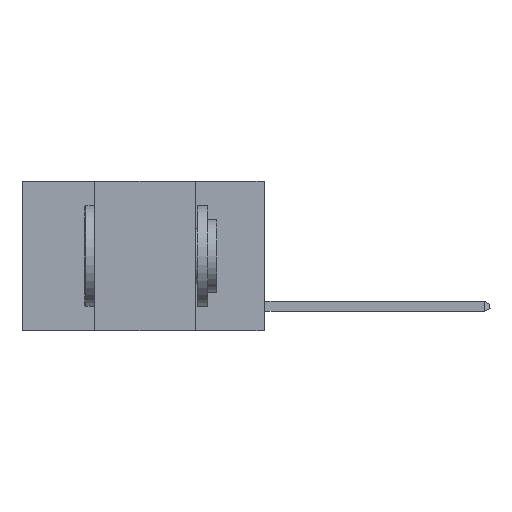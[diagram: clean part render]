
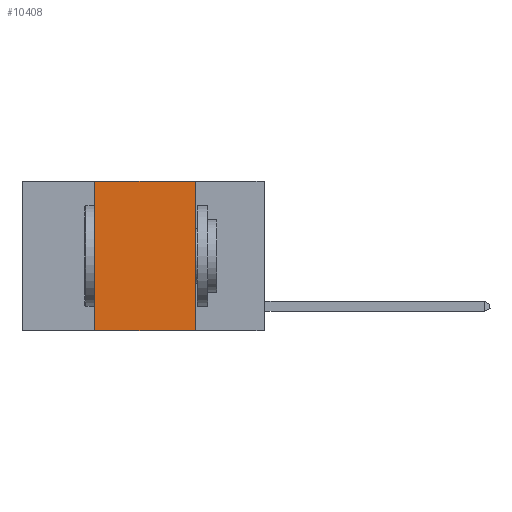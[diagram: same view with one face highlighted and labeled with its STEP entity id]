
A CAD part, left-side view. The second image highlights one B-rep face of the part: STEP entity #10408.
In plain terms, the highlighted planar face has unit normal (-1, 0, 0).
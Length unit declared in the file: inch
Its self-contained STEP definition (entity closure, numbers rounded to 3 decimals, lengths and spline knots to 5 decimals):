
#998 = ORIENTED_EDGE ( 'NONE', *, *, #8480, .F. ) ;
#1108 = DIRECTION ( 'NONE',  ( 0., -1., 0. ) ) ;
#1844 = DIRECTION ( 'NONE',  ( 0., 0., 1. ) ) ;
#1891 = ORIENTED_EDGE ( 'NONE', *, *, #21364, .F. ) ;
#2675 = VERTEX_POINT ( 'NONE', #15466 ) ;
#3230 = CARTESIAN_POINT ( 'NONE',  ( 0., 0.6, 0. ) ) ;
#3592 = VECTOR ( 'NONE', #5515, 39.37008 ) ;
#3967 = ORIENTED_EDGE ( 'NONE', *, *, #22589, .T. ) ;
#4655 = CARTESIAN_POINT ( 'NONE',  ( 0., 0.17, -0.37 ) ) ;
#5374 = VECTOR ( 'NONE', #13527, 39.37008 ) ;
#5515 = DIRECTION ( 'NONE',  ( 0., -1., 0. ) ) ;
#7058 = CARTESIAN_POINT ( 'NONE',  ( 0., 0.6, -0.37 ) ) ;
#7337 = VERTEX_POINT ( 'NONE', #4655 ) ;
#8096 = CARTESIAN_POINT ( 'NONE',  ( 0., 0.42, -0.37 ) ) ;
#8480 = EDGE_CURVE ( 'NONE', #9922, #2675, #15654, .T. ) ;
#9922 = VERTEX_POINT ( 'NONE', #22747 ) ;
#10130 = CARTESIAN_POINT ( 'NONE',  ( 0., 0.6, 0. ) ) ;
#10408 = ADVANCED_FACE ( 'NONE', ( #23073 ), #13921, .F. ) ;
#11454 = VECTOR ( 'NONE', #1844, 39.37008 ) ;
#11644 = LINE ( 'NONE', #13650, #5374 ) ;
#12960 = EDGE_CURVE ( 'NONE', #2675, #7337, #11644, .T. ) ;
#13527 = DIRECTION ( 'NONE',  ( 0., 0., -1. ) ) ;
#13650 = CARTESIAN_POINT ( 'NONE',  ( 0., 0.17, 0. ) ) ;
#13921 = PLANE ( 'NONE',  #17642 ) ;
#14036 = DIRECTION ( 'NONE',  ( 0., 0., -1. ) ) ;
#14252 = CARTESIAN_POINT ( 'NONE',  ( 0., 0.42, 0. ) ) ;
#15466 = CARTESIAN_POINT ( 'NONE',  ( 0., 0.17, 0. ) ) ;
#15654 = LINE ( 'NONE', #3230, #20997 ) ;
#17642 = AXIS2_PLACEMENT_3D ( 'NONE', #10130, #21169, #14036 ) ;
#17941 = ORIENTED_EDGE ( 'NONE', *, *, #12960, .F. ) ;
#18650 = EDGE_LOOP ( 'NONE', ( #17941, #998, #1891, #3967 ) ) ;
#19721 = LINE ( 'NONE', #7058, #3592 ) ;
#20997 = VECTOR ( 'NONE', #1108, 39.37008 ) ;
#21169 = DIRECTION ( 'NONE',  ( 1., 0., 0. ) ) ;
#21364 = EDGE_CURVE ( 'NONE', #22813, #9922, #23175, .T. ) ;
#22589 = EDGE_CURVE ( 'NONE', #22813, #7337, #19721, .T. ) ;
#22747 = CARTESIAN_POINT ( 'NONE',  ( 0., 0.42, 0. ) ) ;
#22813 = VERTEX_POINT ( 'NONE', #8096 ) ;
#23073 = FACE_OUTER_BOUND ( 'NONE', #18650, .T. ) ;
#23175 = LINE ( 'NONE', #14252, #11454 ) ;
